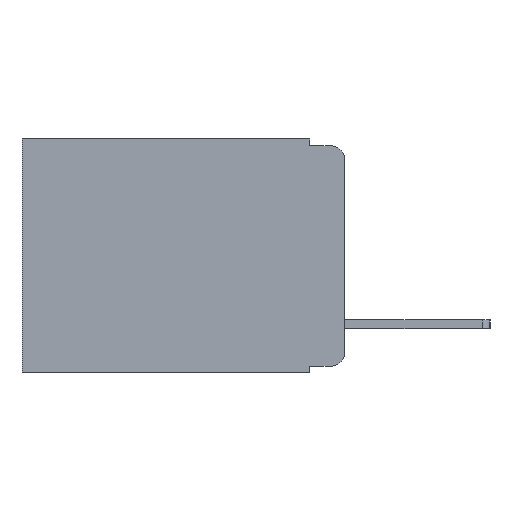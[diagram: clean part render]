
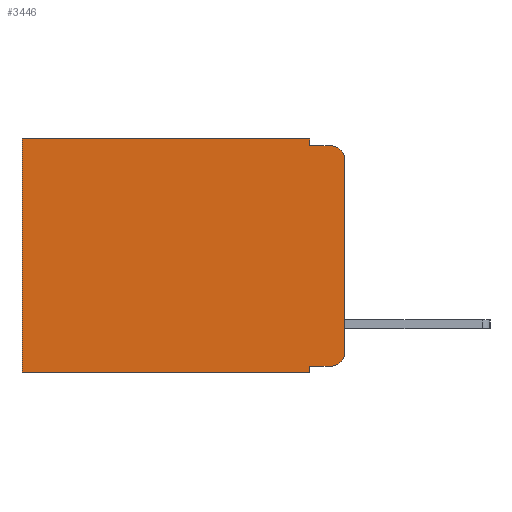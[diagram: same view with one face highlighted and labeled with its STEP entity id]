
A CAD part, left-side view. The second image highlights one B-rep face of the part: STEP entity #3446.
In plain terms, the highlighted planar face has unit normal (-1, 0, 0).
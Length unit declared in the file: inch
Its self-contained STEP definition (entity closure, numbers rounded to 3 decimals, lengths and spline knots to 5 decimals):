
#3 = ORIENTED_EDGE ( 'NONE', *, *, #8922, .F. ) ;
#41 = LINE ( 'NONE', #6152, #12207 ) ;
#46 = CARTESIAN_POINT ( 'NONE',  ( 0.298, 0.051, 0. ) ) ;
#49 = ORIENTED_EDGE ( 'NONE', *, *, #14813, .T. ) ;
#219 = ORIENTED_EDGE ( 'NONE', *, *, #14160, .T. ) ;
#220 = ORIENTED_EDGE ( 'NONE', *, *, #11697, .F. ) ;
#292 = ORIENTED_EDGE ( 'NONE', *, *, #10515, .T. ) ;
#303 = LINE ( 'NONE', #4830, #9280 ) ;
#343 = AXIS2_PLACEMENT_3D ( 'NONE', #3502, #11630, #4809 ) ;
#360 = DIRECTION ( 'NONE',  ( 0., -1., 0. ) ) ;
#459 = CARTESIAN_POINT ( 'NONE',  ( 0.298, 0.051, -0.01 ) ) ;
#573 = VERTEX_POINT ( 'NONE', #46 ) ;
#630 = VERTEX_POINT ( 'NONE', #8004 ) ;
#788 = VERTEX_POINT ( 'NONE', #3270 ) ;
#890 = CARTESIAN_POINT ( 'NONE',  ( 0.298, 0.473, 0. ) ) ;
#1096 = DIRECTION ( 'NONE',  ( 0., 0., -1. ) ) ;
#1364 = CARTESIAN_POINT ( 'NONE',  ( 0.298, 0.473, 0. ) ) ;
#1529 = EDGE_CURVE ( 'NONE', #573, #3811, #9629, .T. ) ;
#1547 = CARTESIAN_POINT ( 'NONE',  ( 0.298, 0.02, -0.03 ) ) ;
#1842 = VECTOR ( 'NONE', #10932, 39.37008 ) ;
#1937 = VECTOR ( 'NONE', #14198, 39.37008 ) ;
#2117 = ORIENTED_EDGE ( 'NONE', *, *, #13916, .F. ) ;
#2307 = ORIENTED_EDGE ( 'NONE', *, *, #11123, .T. ) ;
#2459 = CARTESIAN_POINT ( 'NONE',  ( 0.298, 0.051, 0. ) ) ;
#2668 = CIRCLE ( 'NONE', #343, 0.02 ) ;
#2814 = DIRECTION ( 'NONE',  ( 0., 0., -1. ) ) ;
#2927 = CIRCLE ( 'NONE', #6219, 0.02 ) ;
#3270 = CARTESIAN_POINT ( 'NONE',  ( 0.298, 0., -0.313 ) ) ;
#3446 = ADVANCED_FACE ( 'NONE', ( #14590 ), #5560, .F. ) ;
#3502 = CARTESIAN_POINT ( 'NONE',  ( 0.298, 0.02, -0.313 ) ) ;
#3722 = DIRECTION ( 'NONE',  ( 0., 1., 0. ) ) ;
#3811 = VERTEX_POINT ( 'NONE', #890 ) ;
#3893 = VECTOR ( 'NONE', #1096, 39.37008 ) ;
#4109 = CARTESIAN_POINT ( 'NONE',  ( 0.298, 0., 0. ) ) ;
#4123 = EDGE_LOOP ( 'NONE', ( #220, #49, #8971, #13710, #4963, #2307, #2117, #3, #219, #292 ) ) ;
#4310 = DIRECTION ( 'NONE',  ( 0., 0., -1. ) ) ;
#4434 = CARTESIAN_POINT ( 'NONE',  ( 0.298, 0.051, -0.333 ) ) ;
#4645 = VERTEX_POINT ( 'NONE', #4434 ) ;
#4713 = EDGE_CURVE ( 'NONE', #14092, #10949, #11397, .T. ) ;
#4809 = DIRECTION ( 'NONE',  ( 0., 0., -1. ) ) ;
#4830 = CARTESIAN_POINT ( 'NONE',  ( 0.298, 0., 0. ) ) ;
#4870 = LINE ( 'NONE', #1364, #1842 ) ;
#4963 = ORIENTED_EDGE ( 'NONE', *, *, #1529, .T. ) ;
#5349 = CARTESIAN_POINT ( 'NONE',  ( 0.298, 0.051, -0.333 ) ) ;
#5560 = PLANE ( 'NONE',  #11271 ) ;
#6152 = CARTESIAN_POINT ( 'NONE',  ( 0.298, 0., -0.343 ) ) ;
#6219 = AXIS2_PLACEMENT_3D ( 'NONE', #1547, #10006, #2814 ) ;
#6274 = EDGE_CURVE ( 'NONE', #573, #14092, #13008, .T. ) ;
#6836 = VECTOR ( 'NONE', #360, 39.37008 ) ;
#6977 = DIRECTION ( 'NONE',  ( 0., 0., -1. ) ) ;
#7154 = CARTESIAN_POINT ( 'NONE',  ( 0.298, 0.02, -0.01 ) ) ;
#8004 = CARTESIAN_POINT ( 'NONE',  ( 0.298, 0.02, -0.333 ) ) ;
#8429 = VERTEX_POINT ( 'NONE', #11069 ) ;
#8572 = DIRECTION ( 'NONE',  ( 0., 1., 0. ) ) ;
#8922 = EDGE_CURVE ( 'NONE', #4645, #13135, #14707, .T. ) ;
#8971 = ORIENTED_EDGE ( 'NONE', *, *, #4713, .F. ) ;
#8986 = CARTESIAN_POINT ( 'NONE',  ( 0.298, 0.473, -0.343 ) ) ;
#8992 = DIRECTION ( 'NONE',  ( 1., 0., 0. ) ) ;
#9280 = VECTOR ( 'NONE', #12724, 39.37008 ) ;
#9451 = VERTEX_POINT ( 'NONE', #8986 ) ;
#9629 = LINE ( 'NONE', #4109, #12081 ) ;
#9891 = LINE ( 'NONE', #5349, #6836 ) ;
#10006 = DIRECTION ( 'NONE',  ( -1., 0., 0. ) ) ;
#10285 = CARTESIAN_POINT ( 'NONE',  ( 0.298, 0.051, -0.343 ) ) ;
#10515 = EDGE_CURVE ( 'NONE', #630, #788, #2668, .T. ) ;
#10932 = DIRECTION ( 'NONE',  ( 0., 0., -1. ) ) ;
#10949 = VERTEX_POINT ( 'NONE', #7154 ) ;
#11069 = CARTESIAN_POINT ( 'NONE',  ( 0.298, 0., -0.03 ) ) ;
#11123 = EDGE_CURVE ( 'NONE', #3811, #9451, #4870, .T. ) ;
#11243 = CARTESIAN_POINT ( 'NONE',  ( 0.298, 0.051, 0. ) ) ;
#11271 = AXIS2_PLACEMENT_3D ( 'NONE', #12262, #8992, #6977 ) ;
#11397 = LINE ( 'NONE', #459, #1937 ) ;
#11630 = DIRECTION ( 'NONE',  ( -1., 0., 0. ) ) ;
#11697 = EDGE_CURVE ( 'NONE', #8429, #788, #303, .T. ) ;
#12081 = VECTOR ( 'NONE', #3722, 39.37008 ) ;
#12172 = VECTOR ( 'NONE', #4310, 39.37008 ) ;
#12207 = VECTOR ( 'NONE', #8572, 39.37008 ) ;
#12262 = CARTESIAN_POINT ( 'NONE',  ( 0.298, 0., 0. ) ) ;
#12724 = DIRECTION ( 'NONE',  ( 0., 0., -1. ) ) ;
#13008 = LINE ( 'NONE', #2459, #3893 ) ;
#13135 = VERTEX_POINT ( 'NONE', #10285 ) ;
#13710 = ORIENTED_EDGE ( 'NONE', *, *, #6274, .F. ) ;
#13916 = EDGE_CURVE ( 'NONE', #13135, #9451, #41, .T. ) ;
#14092 = VERTEX_POINT ( 'NONE', #14185 ) ;
#14160 = EDGE_CURVE ( 'NONE', #4645, #630, #9891, .T. ) ;
#14185 = CARTESIAN_POINT ( 'NONE',  ( 0.298, 0.051, -0.01 ) ) ;
#14198 = DIRECTION ( 'NONE',  ( 0., -1., 0. ) ) ;
#14590 = FACE_OUTER_BOUND ( 'NONE', #4123, .T. ) ;
#14707 = LINE ( 'NONE', #11243, #12172 ) ;
#14813 = EDGE_CURVE ( 'NONE', #8429, #10949, #2927, .T. ) ;
